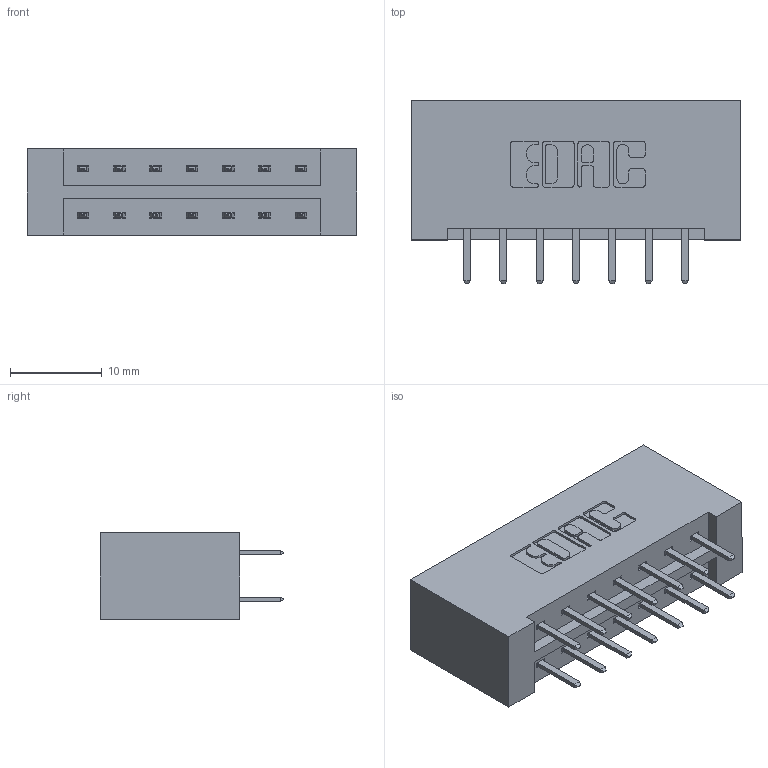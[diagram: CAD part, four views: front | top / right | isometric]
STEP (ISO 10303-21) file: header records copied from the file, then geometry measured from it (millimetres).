
FILE_DESCRIPTION (( 'STEP AP203' ), '1' );
FILE_NAME ('333-014-520-201.STEP', '2018-08-01T01:52:31', ( '' ), ( '' ), 'SwSTEP 2.0', 'SolidWorks 2016', '' );
FILE_SCHEMA (( 'CONFIG_CONTROL_DESIGN' ));
Length unit declared in the file: inch
Products named in the file (3): 333 Part_Lugless; 333-014-520-201; 345-292-001_345-293-120
Assembly tree (15 placements, depth 2):
  333-014-520-201
    333 Part_Lugless
    345-292-001_345-293-120  x14
Bounding box: 35.99 x 20.02 x 9.4 mm (x, y, z)
Volume: 3973.3 mm3; surface area: 4329.4 mm2
Topology: 15 solids, 15 shells, 890 faces, 2569 edges, 1674 vertices
Faces by surface type: plane 598, cylinder 292
Entity records: 8867 total; most frequent: CARTESIAN_POINT 1522, ORIENTED_EDGE 1446, DIRECTION 1343, EDGE_CURVE 723, LINE 599, VECTOR 599, VERTEX_POINT 478, AXIS2_PLACEMENT_3D 372
